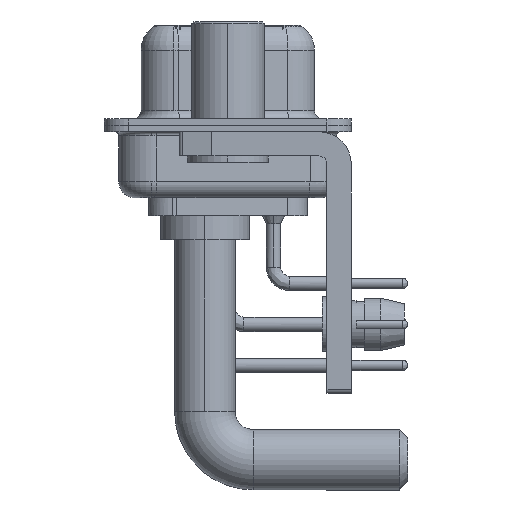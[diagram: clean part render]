
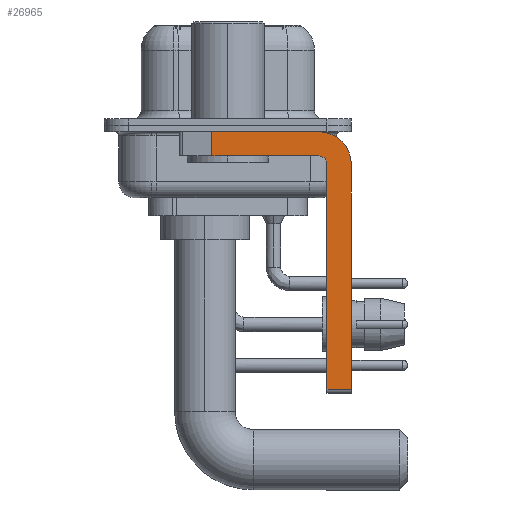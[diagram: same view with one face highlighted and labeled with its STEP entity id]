
A CAD part, left-side view. The second image highlights one B-rep face of the part: STEP entity #26965.
In plain terms, the highlighted planar face has unit normal (-1, 0, 0).
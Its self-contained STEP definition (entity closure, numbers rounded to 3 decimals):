
#768 = DIRECTION ( 'NONE',  ( 0., 0., -1. ) ) ;
#968 = VECTOR ( 'NONE', #3624, 1000. ) ;
#2037 = AXIS2_PLACEMENT_3D ( 'NONE', #12582, #7751, #27893 ) ;
#3143 = VERTEX_POINT ( 'NONE', #15224 ) ;
#3552 = ORIENTED_EDGE ( 'NONE', *, *, #9106, .F. ) ;
#3624 = DIRECTION ( 'NONE',  ( 0., -1., 0. ) ) ;
#5058 = ORIENTED_EDGE ( 'NONE', *, *, #18190, .F. ) ;
#5475 = VERTEX_POINT ( 'NONE', #12632 ) ;
#5913 = LINE ( 'NONE', #24948, #20093 ) ;
#7434 = LINE ( 'NONE', #29577, #24299 ) ;
#7657 = CARTESIAN_POINT ( 'NONE',  ( -2.9, -6.15, -16.6 ) ) ;
#7751 = DIRECTION ( 'NONE',  ( -1., 0., 0. ) ) ;
#8326 = VERTEX_POINT ( 'NONE', #26256 ) ;
#8679 = VERTEX_POINT ( 'NONE', #29980 ) ;
#8691 = VERTEX_POINT ( 'NONE', #25007 ) ;
#9106 = EDGE_CURVE ( 'NONE', #18562, #32450, #25148, .T. ) ;
#9139 = ORIENTED_EDGE ( 'NONE', *, *, #12330, .T. ) ;
#9350 = VECTOR ( 'NONE', #25303, 1000. ) ;
#10088 = DIRECTION ( 'NONE',  ( 0., 1., 0. ) ) ;
#10255 = AXIS2_PLACEMENT_3D ( 'NONE', #13734, #18231, #21206 ) ;
#10532 = CIRCLE ( 'NONE', #2037, 0.5 ) ;
#12330 = EDGE_CURVE ( 'NONE', #18562, #8691, #29067, .T. ) ;
#12576 = EDGE_CURVE ( 'NONE', #32450, #8326, #10532, .T. ) ;
#12582 = CARTESIAN_POINT ( 'NONE',  ( -2.9, -5.65, -2.4 ) ) ;
#12632 = CARTESIAN_POINT ( 'NONE',  ( -2.9, -5.65, -0.4 ) ) ;
#12715 = ORIENTED_EDGE ( 'NONE', *, *, #21552, .T. ) ;
#13206 = ORIENTED_EDGE ( 'NONE', *, *, #31947, .F. ) ;
#13734 = CARTESIAN_POINT ( 'NONE',  ( -2.9, -5.65, -2.4 ) ) ;
#15224 = CARTESIAN_POINT ( 'NONE',  ( -2.9, 0.978, -0.4 ) ) ;
#16013 = LINE ( 'NONE', #30806, #31001 ) ;
#16122 = CARTESIAN_POINT ( 'NONE',  ( -2.9, -7.65, -2.4 ) ) ;
#17201 = DIRECTION ( 'NONE',  ( 0., 0., -1. ) ) ;
#18190 = EDGE_CURVE ( 'NONE', #8326, #8679, #7434, .T. ) ;
#18231 = DIRECTION ( 'NONE',  ( 1., 0., 0. ) ) ;
#18383 = PLANE ( 'NONE',  #10255 ) ;
#18562 = VERTEX_POINT ( 'NONE', #27206 ) ;
#19125 = ORIENTED_EDGE ( 'NONE', *, *, #12576, .F. ) ;
#19294 = VERTEX_POINT ( 'NONE', #16122 ) ;
#20093 = VECTOR ( 'NONE', #768, 1000. ) ;
#21206 = DIRECTION ( 'NONE',  ( 0., 0., -1. ) ) ;
#21552 = EDGE_CURVE ( 'NONE', #3143, #8679, #5913, .T. ) ;
#22019 = DIRECTION ( 'NONE',  ( 1., 0., 0. ) ) ;
#23066 = AXIS2_PLACEMENT_3D ( 'NONE', #24844, #22019, #17201 ) ;
#23535 = ORIENTED_EDGE ( 'NONE', *, *, #24705, .F. ) ;
#23559 = FACE_OUTER_BOUND ( 'NONE', #28830, .T. ) ;
#24299 = VECTOR ( 'NONE', #10088, 1000. ) ;
#24454 = CARTESIAN_POINT ( 'NONE',  ( -2.9, 3., -0.4 ) ) ;
#24705 = EDGE_CURVE ( 'NONE', #3143, #5475, #29903, .T. ) ;
#24844 = CARTESIAN_POINT ( 'NONE',  ( -2.9, -5.65, -2.4 ) ) ;
#24948 = CARTESIAN_POINT ( 'NONE',  ( -2.9, 0.978, -1.9 ) ) ;
#25007 = CARTESIAN_POINT ( 'NONE',  ( -2.9, -7.65, -16.35 ) ) ;
#25148 = LINE ( 'NONE', #7657, #9350 ) ;
#25303 = DIRECTION ( 'NONE',  ( 0., 0., 1. ) ) ;
#25673 = DIRECTION ( 'NONE',  ( 0., 0., -1. ) ) ;
#26256 = CARTESIAN_POINT ( 'NONE',  ( -2.9, -5.65, -1.9 ) ) ;
#26965 = ADVANCED_FACE ( 'NONE', ( #23559 ), #18383, .F. ) ;
#27206 = CARTESIAN_POINT ( 'NONE',  ( -2.9, -6.15, -16.35 ) ) ;
#27311 = CIRCLE ( 'NONE', #23066, 2. ) ;
#27893 = DIRECTION ( 'NONE',  ( 0., 0., 1. ) ) ;
#28830 = EDGE_LOOP ( 'NONE', ( #23535, #12715, #5058, #19125, #3552, #9139, #13206, #29276 ) ) ;
#29067 = LINE ( 'NONE', #31066, #968 ) ;
#29276 = ORIENTED_EDGE ( 'NONE', *, *, #32338, .F. ) ;
#29330 = VECTOR ( 'NONE', #29423, 1000. ) ;
#29423 = DIRECTION ( 'NONE',  ( 0., -1., 0. ) ) ;
#29577 = CARTESIAN_POINT ( 'NONE',  ( -2.9, -5.65, -1.9 ) ) ;
#29903 = LINE ( 'NONE', #24454, #29330 ) ;
#29980 = CARTESIAN_POINT ( 'NONE',  ( -2.9, 0.978, -1.9 ) ) ;
#30806 = CARTESIAN_POINT ( 'NONE',  ( -2.9, -7.65, -2.4 ) ) ;
#31001 = VECTOR ( 'NONE', #25673, 1000. ) ;
#31066 = CARTESIAN_POINT ( 'NONE',  ( -2.9, -5.65, -16.35 ) ) ;
#31947 = EDGE_CURVE ( 'NONE', #19294, #8691, #16013, .T. ) ;
#32163 = CARTESIAN_POINT ( 'NONE',  ( -2.9, -6.15, -2.4 ) ) ;
#32338 = EDGE_CURVE ( 'NONE', #5475, #19294, #27311, .T. ) ;
#32450 = VERTEX_POINT ( 'NONE', #32163 ) ;
